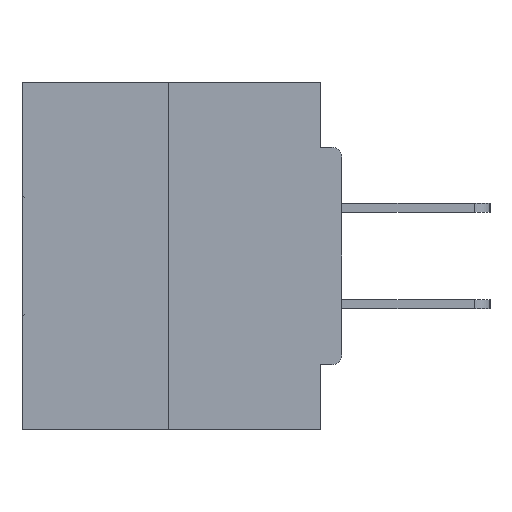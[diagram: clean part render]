
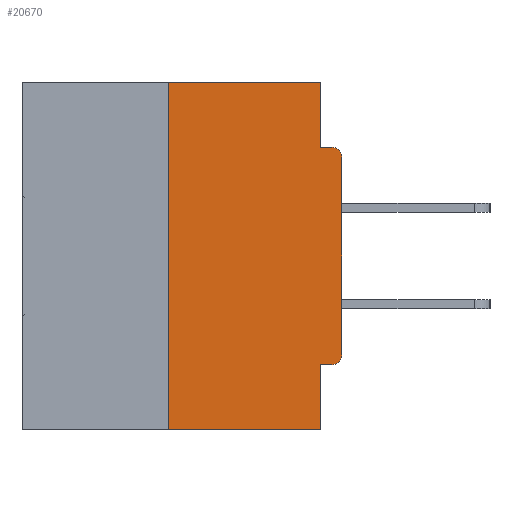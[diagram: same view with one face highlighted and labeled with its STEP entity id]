
A CAD part, left-side view. The second image highlights one B-rep face of the part: STEP entity #20670.
In plain terms, the highlighted planar face has unit normal (-1, 0, 0).
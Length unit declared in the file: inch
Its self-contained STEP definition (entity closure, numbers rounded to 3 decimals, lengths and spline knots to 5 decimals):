
#1190 = VERTEX_POINT ( 'NONE', #18928 ) ;
#1279 = CARTESIAN_POINT ( 'NONE',  ( 0., 0.015, -0.0935 ) ) ;
#1752 = AXIS2_PLACEMENT_3D ( 'NONE', #5378, #24154, #37049 ) ;
#1761 = VERTEX_POINT ( 'NONE', #38784 ) ;
#2462 = VERTEX_POINT ( 'NONE', #1279 ) ;
#2541 = PLANE ( 'NONE',  #40336 ) ;
#2818 = ORIENTED_EDGE ( 'NONE', *, *, #37005, .T. ) ;
#2843 = CARTESIAN_POINT ( 'NONE',  ( 0., 0.031, -0.0935 ) ) ;
#2952 = DIRECTION ( 'NONE',  ( 0., 0., -1. ) ) ;
#3157 = LINE ( 'NONE', #8553, #35663 ) ;
#3733 = ORIENTED_EDGE ( 'NONE', *, *, #31539, .T. ) ;
#4285 = VERTEX_POINT ( 'NONE', #6463 ) ;
#5378 = CARTESIAN_POINT ( 'NONE',  ( 0., 0.015, -0.1085 ) ) ;
#6463 = CARTESIAN_POINT ( 'NONE',  ( 0., 0., -0.3915 ) ) ;
#6866 = AXIS2_PLACEMENT_3D ( 'NONE', #34254, #8918, #34528 ) ;
#6888 = LINE ( 'NONE', #25522, #27103 ) ;
#7039 = FACE_OUTER_BOUND ( 'NONE', #39008, .T. ) ;
#7902 = ORIENTED_EDGE ( 'NONE', *, *, #35032, .F. ) ;
#8379 = DIRECTION ( 'NONE',  ( 0., 0., -1. ) ) ;
#8553 = CARTESIAN_POINT ( 'NONE',  ( 0., 0., 0. ) ) ;
#8918 = DIRECTION ( 'NONE',  ( -1., 0., 0. ) ) ;
#9125 = EDGE_CURVE ( 'NONE', #1190, #17264, #13699, .T. ) ;
#9201 = VECTOR ( 'NONE', #28313, 39.37008 ) ;
#10012 = ORIENTED_EDGE ( 'NONE', *, *, #20924, .F. ) ;
#10992 = ORIENTED_EDGE ( 'NONE', *, *, #9125, .F. ) ;
#11718 = DIRECTION ( 'NONE',  ( 0., 0., 1. ) ) ;
#12818 = DIRECTION ( 'NONE',  ( 0., -1., 0. ) ) ;
#13680 = EDGE_CURVE ( 'NONE', #1761, #20596, #17632, .T. ) ;
#13699 = LINE ( 'NONE', #29798, #34871 ) ;
#14409 = DIRECTION ( 'NONE',  ( 0., -1., 0. ) ) ;
#14531 = EDGE_CURVE ( 'NONE', #17264, #33537, #27917, .T. ) ;
#14596 = VECTOR ( 'NONE', #31219, 39.37008 ) ;
#16974 = LINE ( 'NONE', #33289, #27768 ) ;
#17264 = VERTEX_POINT ( 'NONE', #26495 ) ;
#17389 = VECTOR ( 'NONE', #32120, 39.37008 ) ;
#17538 = CIRCLE ( 'NONE', #6866, 0.015 ) ;
#17632 = LINE ( 'NONE', #25456, #9201 ) ;
#17837 = DIRECTION ( 'NONE',  ( 0., 1., 0. ) ) ;
#18415 = VECTOR ( 'NONE', #8379, 39.37008 ) ;
#18653 = DIRECTION ( 'NONE',  ( 1., 0., 0. ) ) ;
#18928 = CARTESIAN_POINT ( 'NONE',  ( 0., 0.015, -0.4065 ) ) ;
#19120 = CARTESIAN_POINT ( 'NONE',  ( 0., 0.031, -0.5 ) ) ;
#20596 = VERTEX_POINT ( 'NONE', #23910 ) ;
#20670 = ADVANCED_FACE ( 'NONE', ( #7039 ), #2541, .F. ) ;
#20924 = EDGE_CURVE ( 'NONE', #37147, #1761, #25763, .T. ) ;
#22935 = CARTESIAN_POINT ( 'NONE',  ( 0., 0.25, 0. ) ) ;
#23910 = CARTESIAN_POINT ( 'NONE',  ( 0., 0.031, 0. ) ) ;
#24154 = DIRECTION ( 'NONE',  ( -1., 0., 0. ) ) ;
#25456 = CARTESIAN_POINT ( 'NONE',  ( 0., 0.46, 0. ) ) ;
#25522 = CARTESIAN_POINT ( 'NONE',  ( 0., 0., -0.0935 ) ) ;
#25763 = LINE ( 'NONE', #22935, #17389 ) ;
#26075 = CARTESIAN_POINT ( 'NONE',  ( 0., 0., -0.1085 ) ) ;
#26495 = CARTESIAN_POINT ( 'NONE',  ( 0., 0.031, -0.4065 ) ) ;
#27103 = VECTOR ( 'NONE', #12818, 39.37008 ) ;
#27768 = VECTOR ( 'NONE', #14409, 39.37008 ) ;
#27917 = LINE ( 'NONE', #31361, #14596 ) ;
#28313 = DIRECTION ( 'NONE',  ( 0., -1., 0. ) ) ;
#28391 = EDGE_CURVE ( 'NONE', #4285, #31129, #3157, .T. ) ;
#29191 = EDGE_CURVE ( 'NONE', #20596, #39850, #30701, .T. ) ;
#29798 = CARTESIAN_POINT ( 'NONE',  ( 0., 0., -0.4065 ) ) ;
#30677 = CARTESIAN_POINT ( 'NONE',  ( 0., 0.031, 0. ) ) ;
#30701 = LINE ( 'NONE', #30677, #18415 ) ;
#30964 = ORIENTED_EDGE ( 'NONE', *, *, #32114, .T. ) ;
#31129 = VERTEX_POINT ( 'NONE', #26075 ) ;
#31219 = DIRECTION ( 'NONE',  ( 0., 0., -1. ) ) ;
#31321 = CIRCLE ( 'NONE', #1752, 0.015 ) ;
#31361 = CARTESIAN_POINT ( 'NONE',  ( 0., 0.031, -0.5 ) ) ;
#31477 = ORIENTED_EDGE ( 'NONE', *, *, #14531, .F. ) ;
#31539 = EDGE_CURVE ( 'NONE', #1190, #4285, #17538, .T. ) ;
#31600 = ORIENTED_EDGE ( 'NONE', *, *, #13680, .F. ) ;
#32114 = EDGE_CURVE ( 'NONE', #37147, #33537, #16974, .T. ) ;
#32120 = DIRECTION ( 'NONE',  ( 0., 0., 1. ) ) ;
#33289 = CARTESIAN_POINT ( 'NONE',  ( 0., 0.46, -0.5 ) ) ;
#33537 = VERTEX_POINT ( 'NONE', #19120 ) ;
#33865 = ORIENTED_EDGE ( 'NONE', *, *, #28391, .T. ) ;
#34043 = CARTESIAN_POINT ( 'NONE',  ( 0., 0.46, 0. ) ) ;
#34254 = CARTESIAN_POINT ( 'NONE',  ( 0., 0.015, -0.3915 ) ) ;
#34528 = DIRECTION ( 'NONE',  ( 0., 0., -1. ) ) ;
#34871 = VECTOR ( 'NONE', #17837, 39.37008 ) ;
#35032 = EDGE_CURVE ( 'NONE', #39850, #2462, #6888, .T. ) ;
#35524 = CARTESIAN_POINT ( 'NONE',  ( 0., 0.25, -0.5 ) ) ;
#35663 = VECTOR ( 'NONE', #11718, 39.37008 ) ;
#36518 = ORIENTED_EDGE ( 'NONE', *, *, #29191, .F. ) ;
#37005 = EDGE_CURVE ( 'NONE', #31129, #2462, #31321, .T. ) ;
#37049 = DIRECTION ( 'NONE',  ( 0., 0., -1. ) ) ;
#37147 = VERTEX_POINT ( 'NONE', #35524 ) ;
#38784 = CARTESIAN_POINT ( 'NONE',  ( 0., 0.25, 0. ) ) ;
#39008 = EDGE_LOOP ( 'NONE', ( #31600, #10012, #30964, #31477, #10992, #3733, #33865, #2818, #7902, #36518 ) ) ;
#39850 = VERTEX_POINT ( 'NONE', #2843 ) ;
#40336 = AXIS2_PLACEMENT_3D ( 'NONE', #34043, #18653, #2952 ) ;
